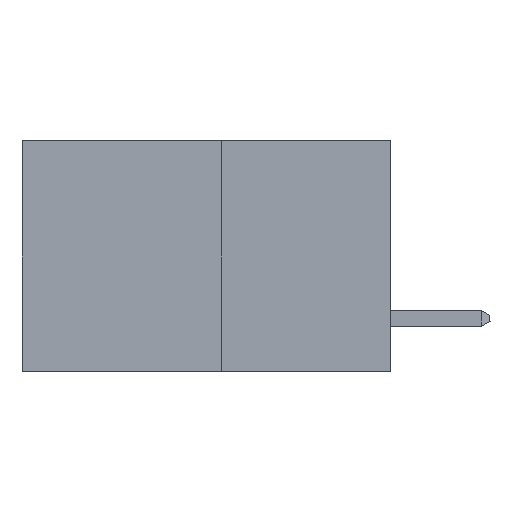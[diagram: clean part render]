
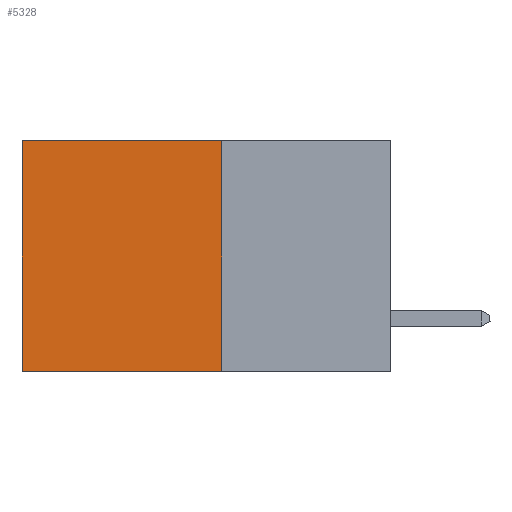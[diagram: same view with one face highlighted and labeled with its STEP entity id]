
A CAD part, left-side view. The second image highlights one B-rep face of the part: STEP entity #5328.
In plain terms, the highlighted planar face has unit normal (-1, 0, 0).
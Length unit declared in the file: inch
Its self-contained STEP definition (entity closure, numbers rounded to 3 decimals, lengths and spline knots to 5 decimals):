
#879 = LINE ( 'NONE', #6593, #13629 ) ;
#1490 = ORIENTED_EDGE ( 'NONE', *, *, #9979, .T. ) ;
#2155 = LINE ( 'NONE', #5481, #14888 ) ;
#2177 = ORIENTED_EDGE ( 'NONE', *, *, #15143, .F. ) ;
#3501 = CARTESIAN_POINT ( 'NONE',  ( 0.277, 0.27, 0. ) ) ;
#3658 = LINE ( 'NONE', #11276, #13104 ) ;
#5328 = ADVANCED_FACE ( 'NONE', ( #9030 ), #10304, .F. ) ;
#5338 = CARTESIAN_POINT ( 'NONE',  ( 0.277, 0.59, -0.37 ) ) ;
#5481 = CARTESIAN_POINT ( 'NONE',  ( 0.277, 0.59, -0.37 ) ) ;
#6593 = CARTESIAN_POINT ( 'NONE',  ( 0.277, 0.27, 0. ) ) ;
#6639 = ORIENTED_EDGE ( 'NONE', *, *, #8113, .T. ) ;
#6731 = CARTESIAN_POINT ( 'NONE',  ( 0.277, 0.59, 0. ) ) ;
#6746 = DIRECTION ( 'NONE',  ( 0., 1., 0. ) ) ;
#7072 = EDGE_CURVE ( 'NONE', #7838, #7665, #3658, .T. ) ;
#7324 = DIRECTION ( 'NONE',  ( 1., 0., 0. ) ) ;
#7394 = CARTESIAN_POINT ( 'NONE',  ( 0.277, 0.27, -0.37 ) ) ;
#7572 = VERTEX_POINT ( 'NONE', #3501 ) ;
#7621 = DIRECTION ( 'NONE',  ( 0., 0., -1. ) ) ;
#7665 = VERTEX_POINT ( 'NONE', #5338 ) ;
#7838 = VERTEX_POINT ( 'NONE', #9346 ) ;
#8113 = EDGE_CURVE ( 'NONE', #7572, #14828, #879, .T. ) ;
#8290 = EDGE_LOOP ( 'NONE', ( #1490, #14379, #2177, #6639 ) ) ;
#8661 = DIRECTION ( 'NONE',  ( 0., 0., -1. ) ) ;
#9030 = FACE_OUTER_BOUND ( 'NONE', #8290, .T. ) ;
#9346 = CARTESIAN_POINT ( 'NONE',  ( 0.277, 0.27, -0.37 ) ) ;
#9979 = EDGE_CURVE ( 'NONE', #14828, #7665, #2155, .T. ) ;
#10304 = PLANE ( 'NONE',  #12980 ) ;
#11175 = DIRECTION ( 'NONE',  ( 0., 1., 0. ) ) ;
#11276 = CARTESIAN_POINT ( 'NONE',  ( 0.277, 0.27, -0.37 ) ) ;
#12275 = LINE ( 'NONE', #7394, #15104 ) ;
#12980 = AXIS2_PLACEMENT_3D ( 'NONE', #14946, #7324, #7621 ) ;
#13104 = VECTOR ( 'NONE', #11175, 39.37008 ) ;
#13629 = VECTOR ( 'NONE', #6746, 39.37008 ) ;
#14379 = ORIENTED_EDGE ( 'NONE', *, *, #7072, .F. ) ;
#14828 = VERTEX_POINT ( 'NONE', #6731 ) ;
#14888 = VECTOR ( 'NONE', #15281, 39.37008 ) ;
#14946 = CARTESIAN_POINT ( 'NONE',  ( 0.277, 0.27, -0.37 ) ) ;
#15104 = VECTOR ( 'NONE', #8661, 39.37008 ) ;
#15143 = EDGE_CURVE ( 'NONE', #7572, #7838, #12275, .T. ) ;
#15281 = DIRECTION ( 'NONE',  ( 0., 0., -1. ) ) ;
